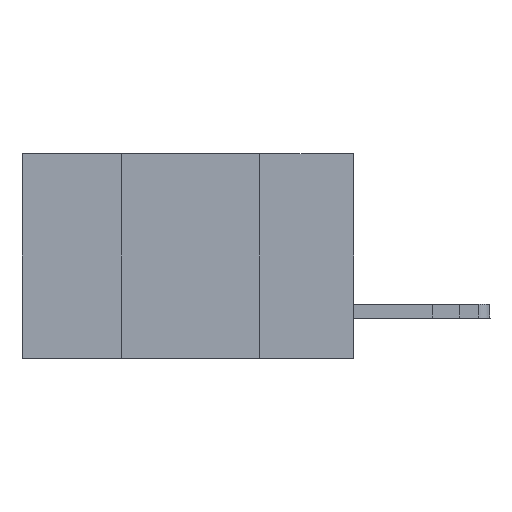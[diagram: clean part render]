
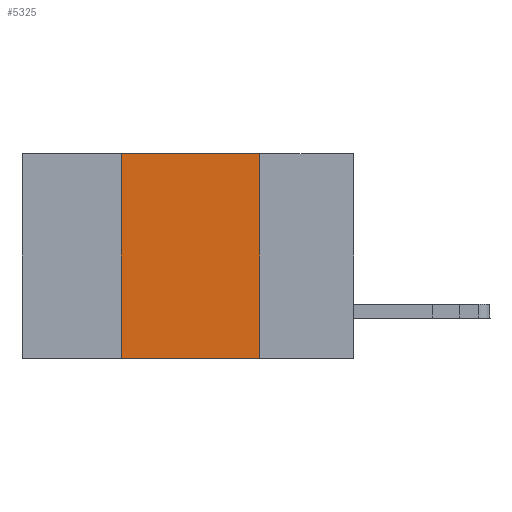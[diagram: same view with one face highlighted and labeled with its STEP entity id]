
A CAD part, left-side view. The second image highlights one B-rep face of the part: STEP entity #5325.
In plain terms, the highlighted planar face has unit normal (-1, 0, 0).
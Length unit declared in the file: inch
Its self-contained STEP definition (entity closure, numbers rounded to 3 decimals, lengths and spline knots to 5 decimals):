
#1951 = EDGE_LOOP ( 'NONE', ( #15157, #25462, #21828, #8322 ) ) ;
#3554 = CARTESIAN_POINT ( 'NONE',  ( 0., 0.42, 0. ) ) ;
#4070 = DIRECTION ( 'NONE',  ( 0., 0., 1. ) ) ;
#4661 = AXIS2_PLACEMENT_3D ( 'NONE', #5395, #19162, #7384 ) ;
#4861 = EDGE_CURVE ( 'NONE', #15284, #11390, #23024, .T. ) ;
#4986 = VECTOR ( 'NONE', #14119, 39.37008 ) ;
#5325 = ADVANCED_FACE ( 'NONE', ( #22390 ), #13302, .F. ) ;
#5395 = CARTESIAN_POINT ( 'NONE',  ( 0., 0.6, 0. ) ) ;
#7384 = DIRECTION ( 'NONE',  ( 0., 0., -1. ) ) ;
#7667 = CARTESIAN_POINT ( 'NONE',  ( 0., 0.42, -0.37 ) ) ;
#7716 = VECTOR ( 'NONE', #25492, 39.37008 ) ;
#8322 = ORIENTED_EDGE ( 'NONE', *, *, #23464, .T. ) ;
#8598 = DIRECTION ( 'NONE',  ( 0., 0., -1. ) ) ;
#9527 = VECTOR ( 'NONE', #8598, 39.37008 ) ;
#11390 = VERTEX_POINT ( 'NONE', #3554 ) ;
#11931 = CARTESIAN_POINT ( 'NONE',  ( 0., 0.6, -0.37 ) ) ;
#12125 = CARTESIAN_POINT ( 'NONE',  ( 0., 0.6, 0. ) ) ;
#13302 = PLANE ( 'NONE',  #4661 ) ;
#14119 = DIRECTION ( 'NONE',  ( 0., -1., 0. ) ) ;
#14587 = CARTESIAN_POINT ( 'NONE',  ( 0., 0.17, 0. ) ) ;
#15157 = ORIENTED_EDGE ( 'NONE', *, *, #24748, .F. ) ;
#15284 = VERTEX_POINT ( 'NONE', #7667 ) ;
#15520 = LINE ( 'NONE', #12125, #4986 ) ;
#16641 = EDGE_CURVE ( 'NONE', #11390, #19557, #15520, .T. ) ;
#19162 = DIRECTION ( 'NONE',  ( 1., 0., 0. ) ) ;
#19487 = CARTESIAN_POINT ( 'NONE',  ( 0., 0.17, -0.37 ) ) ;
#19557 = VERTEX_POINT ( 'NONE', #19598 ) ;
#19598 = CARTESIAN_POINT ( 'NONE',  ( 0., 0.17, 0. ) ) ;
#19785 = CARTESIAN_POINT ( 'NONE',  ( 0., 0.42, 0. ) ) ;
#19975 = LINE ( 'NONE', #14587, #9527 ) ;
#21526 = LINE ( 'NONE', #11931, #7716 ) ;
#21807 = VECTOR ( 'NONE', #4070, 39.37008 ) ;
#21828 = ORIENTED_EDGE ( 'NONE', *, *, #4861, .F. ) ;
#22390 = FACE_OUTER_BOUND ( 'NONE', #1951, .T. ) ;
#23024 = LINE ( 'NONE', #19785, #21807 ) ;
#23464 = EDGE_CURVE ( 'NONE', #15284, #25122, #21526, .T. ) ;
#24748 = EDGE_CURVE ( 'NONE', #19557, #25122, #19975, .T. ) ;
#25122 = VERTEX_POINT ( 'NONE', #19487 ) ;
#25462 = ORIENTED_EDGE ( 'NONE', *, *, #16641, .F. ) ;
#25492 = DIRECTION ( 'NONE',  ( 0., -1., 0. ) ) ;
